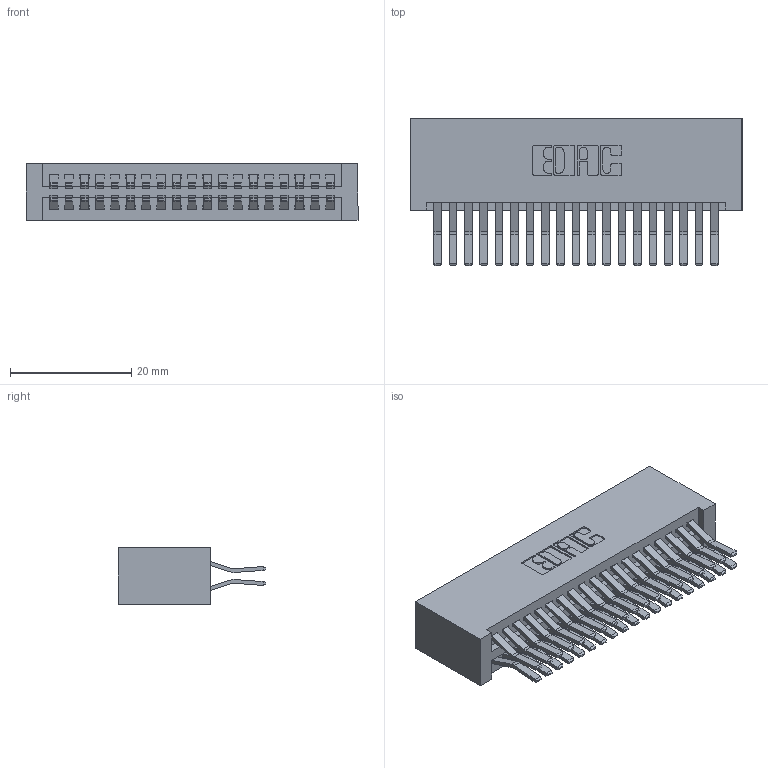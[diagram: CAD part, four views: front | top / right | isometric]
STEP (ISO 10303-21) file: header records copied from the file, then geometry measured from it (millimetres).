
FILE_DESCRIPTION (( 'STEP AP203' ), '1' );
FILE_NAME ('345-038-560-201.STEP', '2018-08-30T10:48:23', ( '' ), ( '' ), 'SwSTEP 2.0', 'SolidWorks 2016', '' );
FILE_SCHEMA (( 'CONFIG_CONTROL_DESIGN' ));
Length unit declared in the file: inch
Products named in the file (3): 345-292-001_560 Tail; 345-038-560-201; 345 Part_No Mounting Lugs
Assembly tree (39 placements, depth 2):
  345-038-560-201
    345 Part_No Mounting Lugs
    345-292-001_560 Tail  x38
Bounding box: 54.86 x 24.45 x 9.4 mm (x, y, z)
Volume: 5981 mm3; surface area: 9339.4 mm2
Topology: 39 solids, 39 shells, 2094 faces, 6207 edges, 4086 vertices
Faces by surface type: plane 1330, cylinder 764
Entity records: 17815 total; most frequent: CARTESIAN_POINT 3008, ORIENTED_EDGE 2942, DIRECTION 2679, EDGE_CURVE 1471, LINE 1267, VECTOR 1267, VERTEX_POINT 978, AXIS2_PLACEMENT_3D 706
